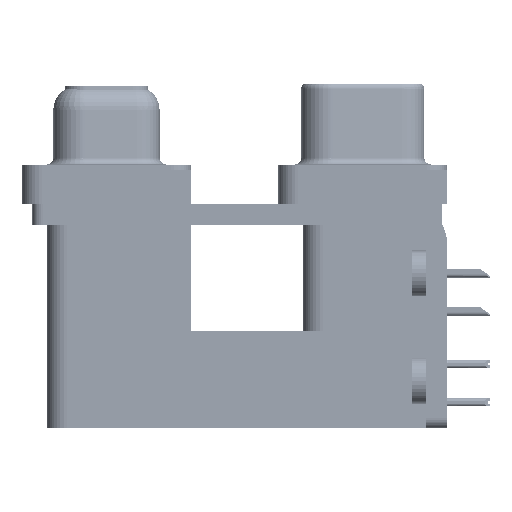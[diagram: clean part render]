
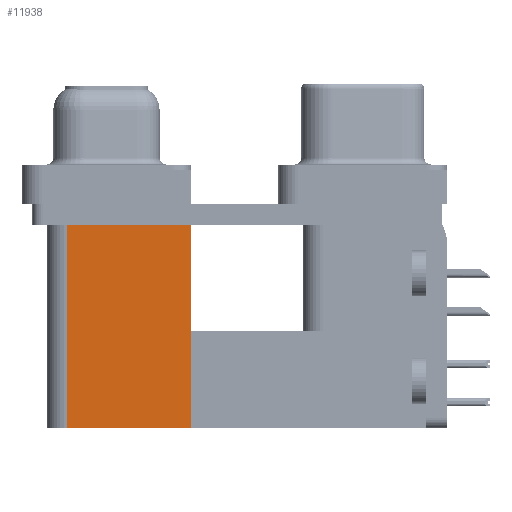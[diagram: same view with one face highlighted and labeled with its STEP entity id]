
A CAD part, left-side view. The second image highlights one B-rep face of the part: STEP entity #11938.
In plain terms, the highlighted planar face has unit normal (-1, 0, 0).
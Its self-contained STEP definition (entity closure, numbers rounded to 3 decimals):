
#583 = ORIENTED_EDGE ( 'NONE', *, *, #50732, .F. ) ;
#2206 = DIRECTION ( 'NONE',  ( 0., 1., 0. ) ) ;
#2467 = DIRECTION ( 'NONE',  ( 0., 1., 0. ) ) ;
#3183 = VERTEX_POINT ( 'NONE', #55643 ) ;
#7350 = DIRECTION ( 'NONE',  ( 0., 1., 0. ) ) ;
#11814 = LINE ( 'NONE', #49171, #66946 ) ;
#11938 = ADVANCED_FACE ( 'NONE', ( #17984 ), #44380, .F. ) ;
#12365 = LINE ( 'NONE', #49020, #38281 ) ;
#14539 = VECTOR ( 'NONE', #2467, 1000. ) ;
#14963 = AXIS2_PLACEMENT_3D ( 'NONE', #65576, #49177, #7350 ) ;
#17550 = CARTESIAN_POINT ( 'NONE',  ( 3.79, 12.775, -2.5 ) ) ;
#17984 = FACE_OUTER_BOUND ( 'NONE', #27422, .T. ) ;
#18832 = VERTEX_POINT ( 'NONE', #29976 ) ;
#18908 = LINE ( 'NONE', #17550, #14539 ) ;
#20276 = ORIENTED_EDGE ( 'NONE', *, *, #37441, .F. ) ;
#27422 = EDGE_LOOP ( 'NONE', ( #50083, #20276, #583, #59924 ) ) ;
#29976 = CARTESIAN_POINT ( 'NONE',  ( 3.79, 21.975, -19.2 ) ) ;
#33405 = EDGE_CURVE ( 'NONE', #46044, #52324, #46149, .T. ) ;
#34699 = CARTESIAN_POINT ( 'NONE',  ( 3.79, 12.775, -2.5 ) ) ;
#35515 = CARTESIAN_POINT ( 'NONE',  ( 3.79, 12.775, -19.2 ) ) ;
#37441 = EDGE_CURVE ( 'NONE', #18832, #3183, #12365, .T. ) ;
#38281 = VECTOR ( 'NONE', #54493, 1000. ) ;
#44380 = PLANE ( 'NONE',  #14963 ) ;
#45545 = VECTOR ( 'NONE', #56396, 1000. ) ;
#46044 = VERTEX_POINT ( 'NONE', #47072 ) ;
#46149 = LINE ( 'NONE', #35515, #45545 ) ;
#47072 = CARTESIAN_POINT ( 'NONE',  ( 3.79, 12.775, -19.2 ) ) ;
#49020 = CARTESIAN_POINT ( 'NONE',  ( 3.79, 21.975, -19.2 ) ) ;
#49171 = CARTESIAN_POINT ( 'NONE',  ( 3.79, 12.775, -19.2 ) ) ;
#49177 = DIRECTION ( 'NONE',  ( 1., 0., 0. ) ) ;
#50083 = ORIENTED_EDGE ( 'NONE', *, *, #53318, .T. ) ;
#50732 = EDGE_CURVE ( 'NONE', #46044, #18832, #11814, .T. ) ;
#52324 = VERTEX_POINT ( 'NONE', #34699 ) ;
#53318 = EDGE_CURVE ( 'NONE', #52324, #3183, #18908, .T. ) ;
#54493 = DIRECTION ( 'NONE',  ( 0., 0., 1. ) ) ;
#55643 = CARTESIAN_POINT ( 'NONE',  ( 3.79, 21.975, -2.5 ) ) ;
#56396 = DIRECTION ( 'NONE',  ( 0., 0., 1. ) ) ;
#59924 = ORIENTED_EDGE ( 'NONE', *, *, #33405, .T. ) ;
#65576 = CARTESIAN_POINT ( 'NONE',  ( 3.79, 12.775, -19.2 ) ) ;
#66946 = VECTOR ( 'NONE', #2206, 1000. ) ;
